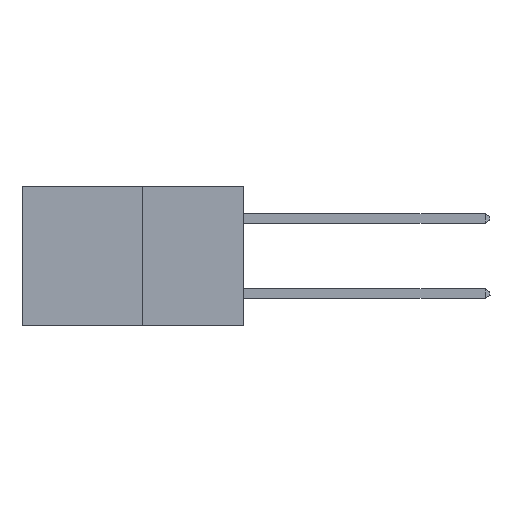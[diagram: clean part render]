
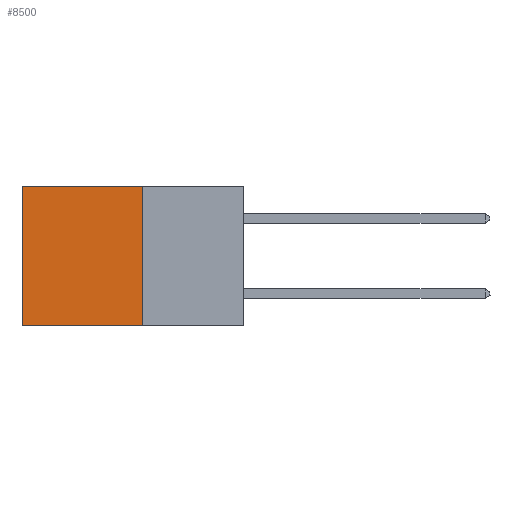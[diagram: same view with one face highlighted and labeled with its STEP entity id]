
A CAD part, left-side view. The second image highlights one B-rep face of the part: STEP entity #8500.
In plain terms, the highlighted planar face has unit normal (-1, 0, 0).
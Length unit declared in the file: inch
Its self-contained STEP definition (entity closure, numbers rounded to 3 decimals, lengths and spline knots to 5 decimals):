
#1211 = EDGE_CURVE ( 'NONE', #11468, #24244, #22646, .T. ) ;
#4503 = DIRECTION ( 'NONE',  ( 0., 1., 0. ) ) ;
#4909 = DIRECTION ( 'NONE',  ( 0., 0., -1. ) ) ;
#7729 = VERTEX_POINT ( 'NONE', #13105 ) ;
#8500 = ADVANCED_FACE ( 'NONE', ( #26711 ), #24898, .F. ) ;
#11105 = CARTESIAN_POINT ( 'NONE',  ( 0.277, 0.59, -0.37 ) ) ;
#11468 = VERTEX_POINT ( 'NONE', #25792 ) ;
#11859 = LINE ( 'NONE', #22599, #23166 ) ;
#12874 = AXIS2_PLACEMENT_3D ( 'NONE', #25003, #23361, #23325 ) ;
#13025 = ORIENTED_EDGE ( 'NONE', *, *, #26551, .F. ) ;
#13105 = CARTESIAN_POINT ( 'NONE',  ( 0.277, 0.27, 0. ) ) ;
#13130 = EDGE_CURVE ( 'NONE', #7729, #22935, #25419, .T. ) ;
#13443 = VECTOR ( 'NONE', #4909, 39.37008 ) ;
#14248 = LINE ( 'NONE', #21554, #25528 ) ;
#14712 = ORIENTED_EDGE ( 'NONE', *, *, #13130, .F. ) ;
#16606 = EDGE_CURVE ( 'NONE', #7729, #11468, #11859, .T. ) ;
#17347 = VECTOR ( 'NONE', #28960, 39.37008 ) ;
#19401 = DIRECTION ( 'NONE',  ( 0., 1., 0. ) ) ;
#21554 = CARTESIAN_POINT ( 'NONE',  ( 0.277, 0.27, -0.37 ) ) ;
#22419 = ORIENTED_EDGE ( 'NONE', *, *, #1211, .T. ) ;
#22599 = CARTESIAN_POINT ( 'NONE',  ( 0.277, 0.27, 0. ) ) ;
#22646 = LINE ( 'NONE', #28989, #17347 ) ;
#22698 = EDGE_LOOP ( 'NONE', ( #22419, #13025, #14712, #23680 ) ) ;
#22935 = VERTEX_POINT ( 'NONE', #26818 ) ;
#22991 = CARTESIAN_POINT ( 'NONE',  ( 0.277, 0.27, -0.37 ) ) ;
#23166 = VECTOR ( 'NONE', #4503, 39.37008 ) ;
#23325 = DIRECTION ( 'NONE',  ( 0., 0., -1. ) ) ;
#23361 = DIRECTION ( 'NONE',  ( 1., 0., 0. ) ) ;
#23680 = ORIENTED_EDGE ( 'NONE', *, *, #16606, .T. ) ;
#24244 = VERTEX_POINT ( 'NONE', #11105 ) ;
#24898 = PLANE ( 'NONE',  #12874 ) ;
#25003 = CARTESIAN_POINT ( 'NONE',  ( 0.277, 0.27, -0.37 ) ) ;
#25419 = LINE ( 'NONE', #22991, #13443 ) ;
#25528 = VECTOR ( 'NONE', #19401, 39.37008 ) ;
#25792 = CARTESIAN_POINT ( 'NONE',  ( 0.277, 0.59, 0. ) ) ;
#26551 = EDGE_CURVE ( 'NONE', #22935, #24244, #14248, .T. ) ;
#26711 = FACE_OUTER_BOUND ( 'NONE', #22698, .T. ) ;
#26818 = CARTESIAN_POINT ( 'NONE',  ( 0.277, 0.27, -0.37 ) ) ;
#28960 = DIRECTION ( 'NONE',  ( 0., 0., -1. ) ) ;
#28989 = CARTESIAN_POINT ( 'NONE',  ( 0.277, 0.59, -0.37 ) ) ;
